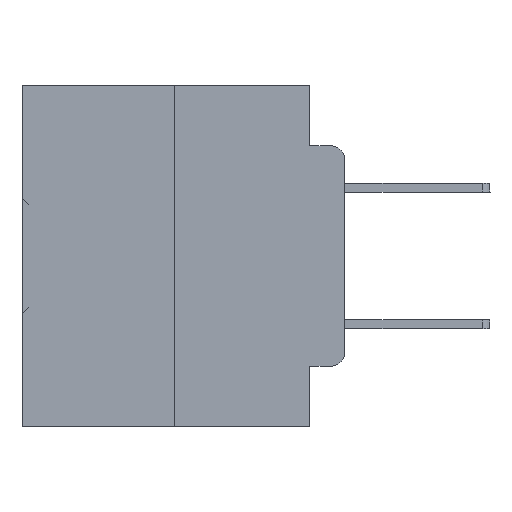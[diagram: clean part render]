
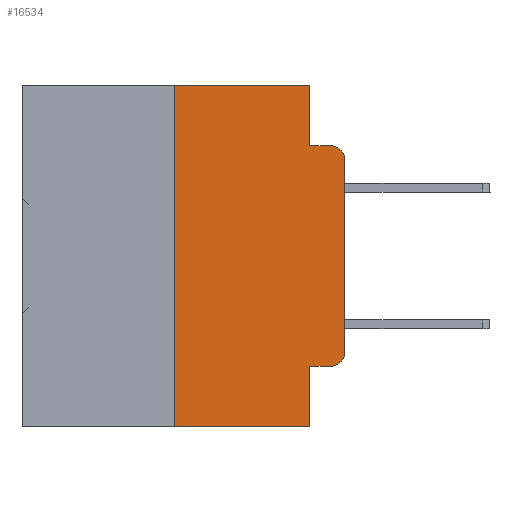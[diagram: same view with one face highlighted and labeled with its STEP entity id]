
A CAD part, left-side view. The second image highlights one B-rep face of the part: STEP entity #16534.
In plain terms, the highlighted planar face has unit normal (-1, 0, 0).
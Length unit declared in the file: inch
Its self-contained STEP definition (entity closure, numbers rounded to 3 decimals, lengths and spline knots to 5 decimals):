
#364 = LINE ( 'NONE', #14782, #4372 ) ;
#750 = CARTESIAN_POINT ( 'NONE',  ( 0., 0.051, -0.5 ) ) ;
#1480 = LINE ( 'NONE', #15886, #11299 ) ;
#1663 = DIRECTION ( 'NONE',  ( 0., -1., 0. ) ) ;
#1705 = LINE ( 'NONE', #12609, #28501 ) ;
#1716 = PLANE ( 'NONE',  #11677 ) ;
#1885 = DIRECTION ( 'NONE',  ( 0., 0., -1. ) ) ;
#1978 = ORIENTED_EDGE ( 'NONE', *, *, #32582, .T. ) ;
#2480 = VERTEX_POINT ( 'NONE', #19522 ) ;
#3164 = CARTESIAN_POINT ( 'NONE',  ( 0., 0.051, 0. ) ) ;
#3545 = CARTESIAN_POINT ( 'NONE',  ( 0., 0.25, -0.5 ) ) ;
#4372 = VECTOR ( 'NONE', #11989, 39.37008 ) ;
#4574 = CARTESIAN_POINT ( 'NONE',  ( 0., 0., -0.3915 ) ) ;
#4900 = VERTEX_POINT ( 'NONE', #30917 ) ;
#5070 = CARTESIAN_POINT ( 'NONE',  ( 0., 0.051, -0.0885 ) ) ;
#6493 = VERTEX_POINT ( 'NONE', #750 ) ;
#6912 = CARTESIAN_POINT ( 'NONE',  ( 0., 0.473, 0. ) ) ;
#7338 = EDGE_LOOP ( 'NONE', ( #10095, #26797, #14741, #12154, #12387, #13541, #8085, #31681, #1978, #31321 ) ) ;
#7636 = CIRCLE ( 'NONE', #33057, 0.02 ) ;
#7666 = DIRECTION ( 'NONE',  ( 0., -1., 0. ) ) ;
#8085 = ORIENTED_EDGE ( 'NONE', *, *, #35378, .T. ) ;
#8446 = DIRECTION ( 'NONE',  ( 0., 0., -1. ) ) ;
#8632 = VERTEX_POINT ( 'NONE', #4574 ) ;
#9757 = DIRECTION ( 'NONE',  ( -1., 0., 0. ) ) ;
#9881 = VERTEX_POINT ( 'NONE', #3164 ) ;
#10004 = VECTOR ( 'NONE', #35473, 39.37008 ) ;
#10095 = ORIENTED_EDGE ( 'NONE', *, *, #29084, .T. ) ;
#10295 = CARTESIAN_POINT ( 'NONE',  ( 0., 0., 0. ) ) ;
#10541 = EDGE_CURVE ( 'NONE', #2480, #9881, #21033, .T. ) ;
#11299 = VECTOR ( 'NONE', #1663, 39.37008 ) ;
#11677 = AXIS2_PLACEMENT_3D ( 'NONE', #6912, #29474, #32820 ) ;
#11852 = LINE ( 'NONE', #26112, #23186 ) ;
#11989 = DIRECTION ( 'NONE',  ( 0., -1., 0. ) ) ;
#12036 = DIRECTION ( 'NONE',  ( 0., 0., -1. ) ) ;
#12154 = ORIENTED_EDGE ( 'NONE', *, *, #32200, .F. ) ;
#12174 = LINE ( 'NONE', #21237, #19416 ) ;
#12387 = ORIENTED_EDGE ( 'NONE', *, *, #10541, .F. ) ;
#12609 = CARTESIAN_POINT ( 'NONE',  ( 0., 0.051, 0. ) ) ;
#13541 = ORIENTED_EDGE ( 'NONE', *, *, #17406, .F. ) ;
#13609 = EDGE_CURVE ( 'NONE', #32409, #26536, #33594, .T. ) ;
#14348 = EDGE_CURVE ( 'NONE', #4900, #8632, #15736, .T. ) ;
#14565 = VECTOR ( 'NONE', #15461, 39.37008 ) ;
#14741 = ORIENTED_EDGE ( 'NONE', *, *, #13609, .F. ) ;
#14782 = CARTESIAN_POINT ( 'NONE',  ( 0., 0.473, -0.5 ) ) ;
#15461 = DIRECTION ( 'NONE',  ( 0., -1., 0. ) ) ;
#15736 = CIRCLE ( 'NONE', #36453, 0.02 ) ;
#15758 = FACE_OUTER_BOUND ( 'NONE', #7338, .T. ) ;
#15886 = CARTESIAN_POINT ( 'NONE',  ( 0., 0.051, -0.4115 ) ) ;
#16123 = CARTESIAN_POINT ( 'NONE',  ( 0., 0., -0.1085 ) ) ;
#16534 = ADVANCED_FACE ( 'NONE', ( #15758 ), #1716, .F. ) ;
#17406 = EDGE_CURVE ( 'NONE', #23664, #2480, #12174, .T. ) ;
#18187 = CARTESIAN_POINT ( 'NONE',  ( 0., 0.051, -0.4115 ) ) ;
#19385 = VECTOR ( 'NONE', #7666, 39.37008 ) ;
#19416 = VECTOR ( 'NONE', #20689, 39.37008 ) ;
#19522 = CARTESIAN_POINT ( 'NONE',  ( 0., 0.25, 0. ) ) ;
#20536 = VERTEX_POINT ( 'NONE', #18187 ) ;
#20689 = DIRECTION ( 'NONE',  ( 0., 0., 1. ) ) ;
#20701 = VERTEX_POINT ( 'NONE', #16123 ) ;
#21033 = LINE ( 'NONE', #26394, #14565 ) ;
#21237 = CARTESIAN_POINT ( 'NONE',  ( 0., 0.25, 0. ) ) ;
#21402 = CARTESIAN_POINT ( 'NONE',  ( 0., 0.02, -0.3915 ) ) ;
#23186 = VECTOR ( 'NONE', #12036, 39.37008 ) ;
#23553 = EDGE_CURVE ( 'NONE', #20536, #6493, #11852, .T. ) ;
#23664 = VERTEX_POINT ( 'NONE', #3545 ) ;
#23748 = CARTESIAN_POINT ( 'NONE',  ( 0., 0.02, -0.0885 ) ) ;
#26112 = CARTESIAN_POINT ( 'NONE',  ( 0., 0.051, 0. ) ) ;
#26394 = CARTESIAN_POINT ( 'NONE',  ( 0., 0.473, 0. ) ) ;
#26536 = VERTEX_POINT ( 'NONE', #23748 ) ;
#26797 = ORIENTED_EDGE ( 'NONE', *, *, #29185, .T. ) ;
#28501 = VECTOR ( 'NONE', #1885, 39.37008 ) ;
#29084 = EDGE_CURVE ( 'NONE', #8632, #20701, #33073, .T. ) ;
#29185 = EDGE_CURVE ( 'NONE', #20701, #26536, #7636, .T. ) ;
#29474 = DIRECTION ( 'NONE',  ( 1., 0., 0. ) ) ;
#30845 = CARTESIAN_POINT ( 'NONE',  ( 0., 0.02, -0.1085 ) ) ;
#30917 = CARTESIAN_POINT ( 'NONE',  ( 0., 0.02, -0.4115 ) ) ;
#31321 = ORIENTED_EDGE ( 'NONE', *, *, #14348, .T. ) ;
#31681 = ORIENTED_EDGE ( 'NONE', *, *, #23553, .F. ) ;
#32200 = EDGE_CURVE ( 'NONE', #9881, #32409, #1705, .T. ) ;
#32409 = VERTEX_POINT ( 'NONE', #33724 ) ;
#32582 = EDGE_CURVE ( 'NONE', #20536, #4900, #1480, .T. ) ;
#32704 = DIRECTION ( 'NONE',  ( 0., 0., -1. ) ) ;
#32820 = DIRECTION ( 'NONE',  ( 0., 0., -1. ) ) ;
#33057 = AXIS2_PLACEMENT_3D ( 'NONE', #30845, #33637, #8446 ) ;
#33073 = LINE ( 'NONE', #10295, #10004 ) ;
#33594 = LINE ( 'NONE', #5070, #19385 ) ;
#33637 = DIRECTION ( 'NONE',  ( -1., 0., 0. ) ) ;
#33724 = CARTESIAN_POINT ( 'NONE',  ( 0., 0.051, -0.0885 ) ) ;
#35378 = EDGE_CURVE ( 'NONE', #23664, #6493, #364, .T. ) ;
#35473 = DIRECTION ( 'NONE',  ( 0., 0., 1. ) ) ;
#36453 = AXIS2_PLACEMENT_3D ( 'NONE', #21402, #9757, #32704 ) ;
